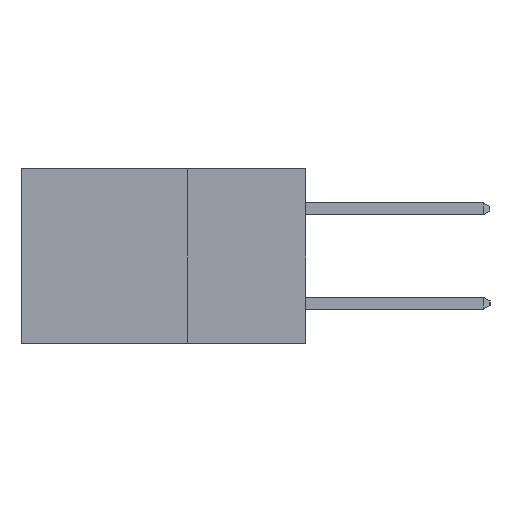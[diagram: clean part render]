
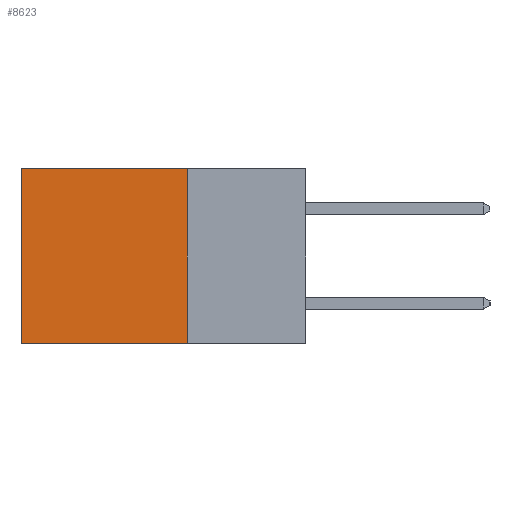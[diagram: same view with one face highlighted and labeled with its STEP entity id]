
A CAD part, left-side view. The second image highlights one B-rep face of the part: STEP entity #8623.
In plain terms, the highlighted planar face has unit normal (-1, 0, 0).
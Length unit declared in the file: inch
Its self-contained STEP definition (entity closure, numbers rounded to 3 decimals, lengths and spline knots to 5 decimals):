
#558 = LINE ( 'NONE', #11980, #8112 ) ;
#587 = CARTESIAN_POINT ( 'NONE',  ( 0.2615, 0.25, -0.37 ) ) ;
#1109 = VERTEX_POINT ( 'NONE', #6352 ) ;
#1210 = ORIENTED_EDGE ( 'NONE', *, *, #8720, .F. ) ;
#2249 = PLANE ( 'NONE',  #5420 ) ;
#2308 = FACE_OUTER_BOUND ( 'NONE', #10656, .T. ) ;
#2719 = VERTEX_POINT ( 'NONE', #13170 ) ;
#3552 = VERTEX_POINT ( 'NONE', #9743 ) ;
#3710 = DIRECTION ( 'NONE',  ( 1., 0., 0. ) ) ;
#3851 = VECTOR ( 'NONE', #17866, 39.37008 ) ;
#4279 = DIRECTION ( 'NONE',  ( 0., 0., -1. ) ) ;
#4719 = DIRECTION ( 'NONE',  ( 0., 0., -1. ) ) ;
#5420 = AXIS2_PLACEMENT_3D ( 'NONE', #587, #3710, #13861 ) ;
#6352 = CARTESIAN_POINT ( 'NONE',  ( 0.2615, 0.25, 0. ) ) ;
#6780 = CARTESIAN_POINT ( 'NONE',  ( 0.2615, 0.25, -0.37 ) ) ;
#8000 = CARTESIAN_POINT ( 'NONE',  ( 0.2615, 0.25, 0. ) ) ;
#8112 = VECTOR ( 'NONE', #4719, 39.37008 ) ;
#8623 = ADVANCED_FACE ( 'NONE', ( #2308 ), #2249, .F. ) ;
#8720 = EDGE_CURVE ( 'NONE', #2719, #3552, #16295, .T. ) ;
#8758 = VECTOR ( 'NONE', #14029, 39.37008 ) ;
#8825 = ORIENTED_EDGE ( 'NONE', *, *, #15138, .F. ) ;
#9400 = ORIENTED_EDGE ( 'NONE', *, *, #10671, .T. ) ;
#9743 = CARTESIAN_POINT ( 'NONE',  ( 0.2615, 0.6, -0.37 ) ) ;
#9839 = CARTESIAN_POINT ( 'NONE',  ( 0.2615, 0.6, 0. ) ) ;
#10656 = EDGE_LOOP ( 'NONE', ( #9400, #1210, #8825, #18065 ) ) ;
#10671 = EDGE_CURVE ( 'NONE', #15716, #3552, #558, .T. ) ;
#11980 = CARTESIAN_POINT ( 'NONE',  ( 0.2615, 0.6, -0.37 ) ) ;
#12845 = LINE ( 'NONE', #15730, #17007 ) ;
#13170 = CARTESIAN_POINT ( 'NONE',  ( 0.2615, 0.25, -0.37 ) ) ;
#13861 = DIRECTION ( 'NONE',  ( 0., 0., -1. ) ) ;
#14029 = DIRECTION ( 'NONE',  ( 0., 1., 0. ) ) ;
#15138 = EDGE_CURVE ( 'NONE', #1109, #2719, #12845, .T. ) ;
#15356 = LINE ( 'NONE', #8000, #3851 ) ;
#15716 = VERTEX_POINT ( 'NONE', #9839 ) ;
#15730 = CARTESIAN_POINT ( 'NONE',  ( 0.2615, 0.25, -0.37 ) ) ;
#16295 = LINE ( 'NONE', #6780, #8758 ) ;
#17007 = VECTOR ( 'NONE', #4279, 39.37008 ) ;
#17512 = EDGE_CURVE ( 'NONE', #1109, #15716, #15356, .T. ) ;
#17866 = DIRECTION ( 'NONE',  ( 0., 1., 0. ) ) ;
#18065 = ORIENTED_EDGE ( 'NONE', *, *, #17512, .T. ) ;
